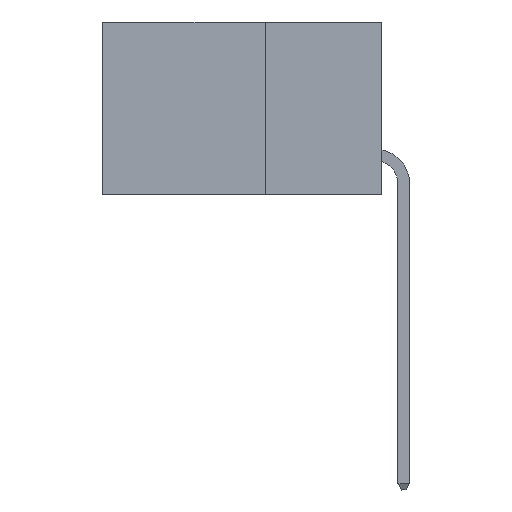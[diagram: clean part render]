
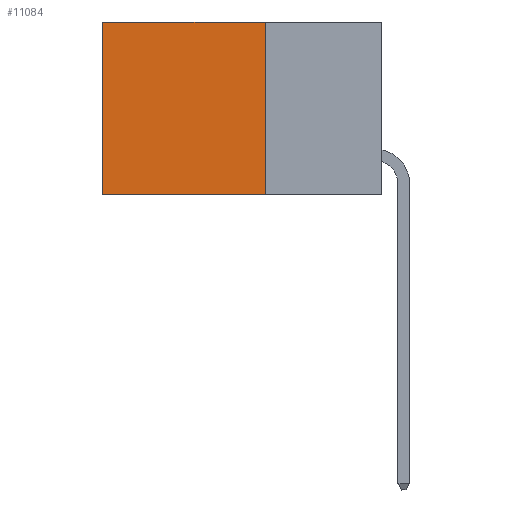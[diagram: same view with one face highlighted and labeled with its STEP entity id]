
A CAD part, left-side view. The second image highlights one B-rep face of the part: STEP entity #11084.
In plain terms, the highlighted planar face has unit normal (-1, 0, 0).
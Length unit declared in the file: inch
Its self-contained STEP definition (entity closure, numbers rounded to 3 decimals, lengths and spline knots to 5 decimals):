
#1785 = CARTESIAN_POINT ( 'NONE',  ( 0.2875, 0.25, 0. ) ) ;
#3138 = CARTESIAN_POINT ( 'NONE',  ( 0.2875, 0.25, 0. ) ) ;
#3462 = VECTOR ( 'NONE', #25357, 39.37008 ) ;
#4061 = VECTOR ( 'NONE', #32165, 39.37008 ) ;
#5097 = EDGE_LOOP ( 'NONE', ( #28074, #9156, #5767, #31834 ) ) ;
#5436 = VERTEX_POINT ( 'NONE', #6000 ) ;
#5767 = ORIENTED_EDGE ( 'NONE', *, *, #12495, .F. ) ;
#6000 = CARTESIAN_POINT ( 'NONE',  ( 0.2875, 0.25, -0.37 ) ) ;
#6081 = EDGE_CURVE ( 'NONE', #35421, #14323, #21415, .T. ) ;
#6125 = CARTESIAN_POINT ( 'NONE',  ( 0.2875, 0.25, 0. ) ) ;
#8630 = AXIS2_PLACEMENT_3D ( 'NONE', #1785, #20623, #14546 ) ;
#9156 = ORIENTED_EDGE ( 'NONE', *, *, #18946, .F. ) ;
#10393 = CARTESIAN_POINT ( 'NONE',  ( 0.2875, 0.6, -0.37 ) ) ;
#11084 = ADVANCED_FACE ( 'NONE', ( #29641 ), #26848, .F. ) ;
#12016 = VECTOR ( 'NONE', #39748, 39.37008 ) ;
#12495 = EDGE_CURVE ( 'NONE', #35421, #5436, #14410, .T. ) ;
#13334 = CARTESIAN_POINT ( 'NONE',  ( 0.2875, 0.25, -0.37 ) ) ;
#14323 = VERTEX_POINT ( 'NONE', #35320 ) ;
#14410 = LINE ( 'NONE', #3138, #3462 ) ;
#14546 = DIRECTION ( 'NONE',  ( 0., 0., -1. ) ) ;
#15938 = LINE ( 'NONE', #26394, #4061 ) ;
#18946 = EDGE_CURVE ( 'NONE', #5436, #31216, #34972, .T. ) ;
#20623 = DIRECTION ( 'NONE',  ( 1., 0., 0. ) ) ;
#21415 = LINE ( 'NONE', #36614, #12016 ) ;
#25357 = DIRECTION ( 'NONE',  ( 0., 0., -1. ) ) ;
#26394 = CARTESIAN_POINT ( 'NONE',  ( 0.2875, 0.6, 0. ) ) ;
#26848 = PLANE ( 'NONE',  #8630 ) ;
#28074 = ORIENTED_EDGE ( 'NONE', *, *, #38607, .T. ) ;
#29641 = FACE_OUTER_BOUND ( 'NONE', #5097, .T. ) ;
#31216 = VERTEX_POINT ( 'NONE', #10393 ) ;
#31834 = ORIENTED_EDGE ( 'NONE', *, *, #6081, .T. ) ;
#32165 = DIRECTION ( 'NONE',  ( 0., 0., -1. ) ) ;
#32511 = VECTOR ( 'NONE', #35529, 39.37008 ) ;
#34972 = LINE ( 'NONE', #13334, #32511 ) ;
#35320 = CARTESIAN_POINT ( 'NONE',  ( 0.2875, 0.6, 0. ) ) ;
#35421 = VERTEX_POINT ( 'NONE', #6125 ) ;
#35529 = DIRECTION ( 'NONE',  ( 0., 1., 0. ) ) ;
#36614 = CARTESIAN_POINT ( 'NONE',  ( 0.2875, 0.25, 0. ) ) ;
#38607 = EDGE_CURVE ( 'NONE', #14323, #31216, #15938, .T. ) ;
#39748 = DIRECTION ( 'NONE',  ( 0., 1., 0. ) ) ;
